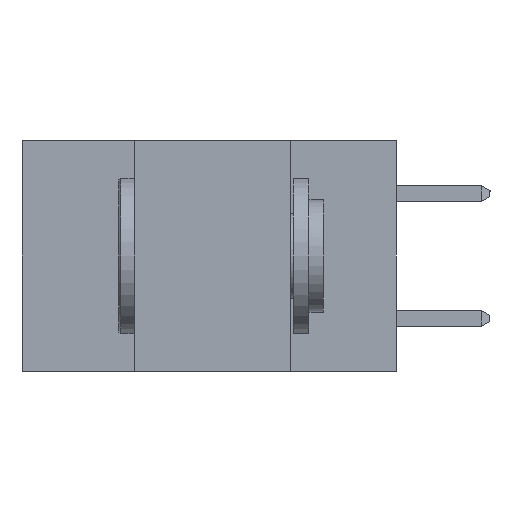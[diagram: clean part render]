
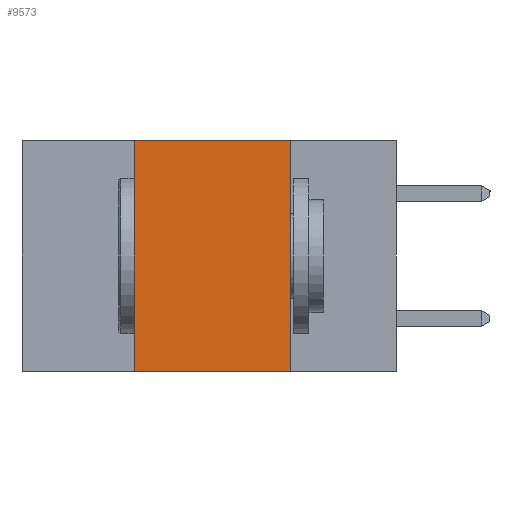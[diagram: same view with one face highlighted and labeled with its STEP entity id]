
A CAD part, left-side view. The second image highlights one B-rep face of the part: STEP entity #9573.
In plain terms, the highlighted planar face has unit normal (-1, 0, 0).
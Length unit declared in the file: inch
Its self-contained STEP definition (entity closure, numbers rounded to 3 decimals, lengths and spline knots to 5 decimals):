
#38 = VERTEX_POINT ( 'NONE', #21731 ) ;
#409 = CARTESIAN_POINT ( 'NONE',  ( 0., 0.17, -0.37 ) ) ;
#487 = AXIS2_PLACEMENT_3D ( 'NONE', #13468, #11892, #3372 ) ;
#3372 = DIRECTION ( 'NONE',  ( 0., 0., -1. ) ) ;
#3947 = EDGE_LOOP ( 'NONE', ( #8283, #3997, #13460, #12878 ) ) ;
#3997 = ORIENTED_EDGE ( 'NONE', *, *, #11484, .F. ) ;
#4362 = VERTEX_POINT ( 'NONE', #409 ) ;
#4973 = DIRECTION ( 'NONE',  ( 0., 0., 1. ) ) ;
#6731 = EDGE_CURVE ( 'NONE', #10652, #15473, #20352, .T. ) ;
#7527 = CARTESIAN_POINT ( 'NONE',  ( 0., 0.17, -0.37 ) ) ;
#8283 = ORIENTED_EDGE ( 'NONE', *, *, #20670, .F. ) ;
#8323 = FACE_OUTER_BOUND ( 'NONE', #3947, .T. ) ;
#9299 = VECTOR ( 'NONE', #12570, 39.37008 ) ;
#9573 = ADVANCED_FACE ( 'NONE', ( #8323 ), #22033, .F. ) ;
#10652 = VERTEX_POINT ( 'NONE', #14805 ) ;
#11484 = EDGE_CURVE ( 'NONE', #15473, #38, #13976, .T. ) ;
#11663 = VECTOR ( 'NONE', #12169, 39.37008 ) ;
#11892 = DIRECTION ( 'NONE',  ( 1., 0., 0. ) ) ;
#12169 = DIRECTION ( 'NONE',  ( 0., -1., 0. ) ) ;
#12378 = VECTOR ( 'NONE', #21496, 39.37008 ) ;
#12570 = DIRECTION ( 'NONE',  ( 0., 0., -1. ) ) ;
#12878 = ORIENTED_EDGE ( 'NONE', *, *, #14531, .T. ) ;
#13460 = ORIENTED_EDGE ( 'NONE', *, *, #6731, .F. ) ;
#13468 = CARTESIAN_POINT ( 'NONE',  ( 0., 0.6, 0. ) ) ;
#13976 = LINE ( 'NONE', #15560, #11663 ) ;
#14531 = EDGE_CURVE ( 'NONE', #10652, #4362, #15977, .T. ) ;
#14805 = CARTESIAN_POINT ( 'NONE',  ( 0., 0.42, -0.37 ) ) ;
#14891 = CARTESIAN_POINT ( 'NONE',  ( 0., 0.42, 0. ) ) ;
#15473 = VERTEX_POINT ( 'NONE', #14891 ) ;
#15560 = CARTESIAN_POINT ( 'NONE',  ( 0., 0.6, 0. ) ) ;
#15977 = LINE ( 'NONE', #18231, #12378 ) ;
#17688 = VECTOR ( 'NONE', #4973, 39.37008 ) ;
#18231 = CARTESIAN_POINT ( 'NONE',  ( 0., 0.6, -0.37 ) ) ;
#18554 = CARTESIAN_POINT ( 'NONE',  ( 0., 0.42, -0.37 ) ) ;
#20352 = LINE ( 'NONE', #18554, #17688 ) ;
#20670 = EDGE_CURVE ( 'NONE', #38, #4362, #21110, .T. ) ;
#21110 = LINE ( 'NONE', #7527, #9299 ) ;
#21496 = DIRECTION ( 'NONE',  ( 0., -1., 0. ) ) ;
#21731 = CARTESIAN_POINT ( 'NONE',  ( 0., 0.17, 0. ) ) ;
#22033 = PLANE ( 'NONE',  #487 ) ;
